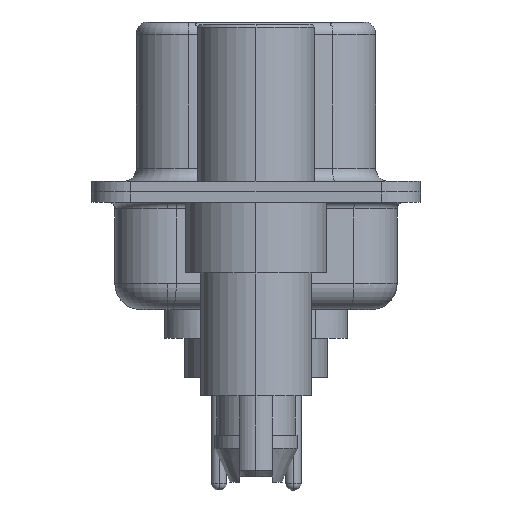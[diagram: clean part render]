
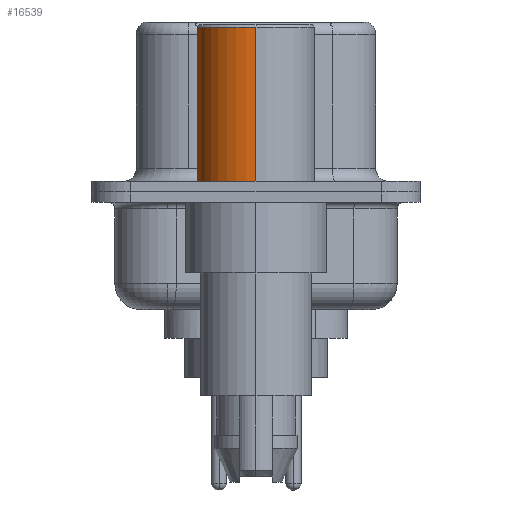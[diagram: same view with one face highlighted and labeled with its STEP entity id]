
A CAD part, left-side view. The second image highlights one B-rep face of the part: STEP entity #16539.
In plain terms, the highlighted cylindrical face has radius 2.25 mm (diameter 4.5 mm), a partial arc.
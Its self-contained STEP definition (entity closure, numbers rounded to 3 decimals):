
#72 = ORIENTED_EDGE ( 'NONE', *, *, #6502, .T. ) ;
#172 = CARTESIAN_POINT ( 'NONE',  ( -2.25, 0., 0.4 ) ) ;
#1216 = CARTESIAN_POINT ( 'NONE',  ( 0., 0., 0.4 ) ) ;
#1352 = CYLINDRICAL_SURFACE ( 'NONE', #12083, 2.25 ) ;
#1649 = ORIENTED_EDGE ( 'NONE', *, *, #20989, .F. ) ;
#4204 = CARTESIAN_POINT ( 'NONE',  ( 2.25, 0., 0.4 ) ) ;
#5473 = LINE ( 'NONE', #19244, #14595 ) ;
#6239 = CIRCLE ( 'NONE', #11236, 2.25 ) ;
#6306 = DIRECTION ( 'NONE',  ( 0., 0., 1. ) ) ;
#6357 = DIRECTION ( 'NONE',  ( 1., 0., 0. ) ) ;
#6502 = EDGE_CURVE ( 'NONE', #12013, #12700, #6239, .T. ) ;
#7117 = VERTEX_POINT ( 'NONE', #9965 ) ;
#7516 = LINE ( 'NONE', #8930, #12773 ) ;
#8407 = DIRECTION ( 'NONE',  ( 1., 0., 0. ) ) ;
#8930 = CARTESIAN_POINT ( 'NONE',  ( 2.25, 0., 0.581 ) ) ;
#9369 = FACE_OUTER_BOUND ( 'NONE', #9388, .T. ) ;
#9388 = EDGE_LOOP ( 'NONE', ( #72, #19598, #16902, #1649 ) ) ;
#9965 = CARTESIAN_POINT ( 'NONE',  ( -2.25, 0., 6.3 ) ) ;
#11193 = CIRCLE ( 'NONE', #16052, 2.25 ) ;
#11236 = AXIS2_PLACEMENT_3D ( 'NONE', #1216, #6306, #8407 ) ;
#12013 = VERTEX_POINT ( 'NONE', #4204 ) ;
#12083 = AXIS2_PLACEMENT_3D ( 'NONE', #17528, #17684, #19672 ) ;
#12700 = VERTEX_POINT ( 'NONE', #172 ) ;
#12773 = VECTOR ( 'NONE', #14494, 1000. ) ;
#14494 = DIRECTION ( 'NONE',  ( 0., 0., 1. ) ) ;
#14595 = VECTOR ( 'NONE', #19466, 1000. ) ;
#15374 = EDGE_CURVE ( 'NONE', #19291, #7117, #11193, .T. ) ;
#16052 = AXIS2_PLACEMENT_3D ( 'NONE', #16878, #22121, #6357 ) ;
#16539 = ADVANCED_FACE ( 'NONE', ( #9369 ), #1352, .T. ) ;
#16878 = CARTESIAN_POINT ( 'NONE',  ( 0., 0., 6.3 ) ) ;
#16902 = ORIENTED_EDGE ( 'NONE', *, *, #15374, .F. ) ;
#17528 = CARTESIAN_POINT ( 'NONE',  ( 0., 0., 0.581 ) ) ;
#17684 = DIRECTION ( 'NONE',  ( 0., 0., 1. ) ) ;
#18170 = CARTESIAN_POINT ( 'NONE',  ( 2.25, 0., 6.3 ) ) ;
#19244 = CARTESIAN_POINT ( 'NONE',  ( -2.25, 0., 0.581 ) ) ;
#19291 = VERTEX_POINT ( 'NONE', #18170 ) ;
#19466 = DIRECTION ( 'NONE',  ( 0., 0., 1. ) ) ;
#19598 = ORIENTED_EDGE ( 'NONE', *, *, #21729, .T. ) ;
#19672 = DIRECTION ( 'NONE',  ( 1., 0., 0. ) ) ;
#20989 = EDGE_CURVE ( 'NONE', #12013, #19291, #7516, .T. ) ;
#21729 = EDGE_CURVE ( 'NONE', #12700, #7117, #5473, .T. ) ;
#22121 = DIRECTION ( 'NONE',  ( 0., 0., 1. ) ) ;
